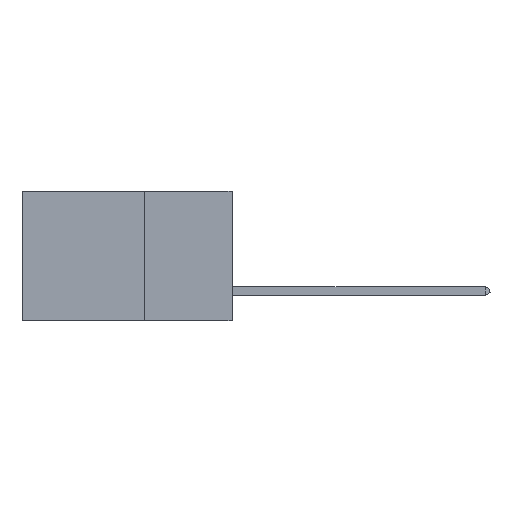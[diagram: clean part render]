
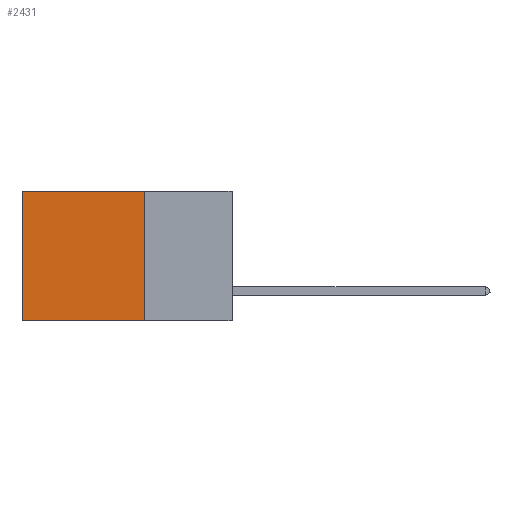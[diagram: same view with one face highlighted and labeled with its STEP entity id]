
A CAD part, left-side view. The second image highlights one B-rep face of the part: STEP entity #2431.
In plain terms, the highlighted planar face has unit normal (-1, 0, 0).
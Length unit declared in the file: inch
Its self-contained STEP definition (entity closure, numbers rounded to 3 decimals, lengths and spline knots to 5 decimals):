
#384 = LINE ( 'NONE', #13258, #7812 ) ;
#436 = CARTESIAN_POINT ( 'NONE',  ( 0.2875, 0.6, 0. ) ) ;
#698 = EDGE_CURVE ( 'NONE', #13443, #2235, #7849, .T. ) ;
#1500 = LINE ( 'NONE', #10485, #12628 ) ;
#2235 = VERTEX_POINT ( 'NONE', #7699 ) ;
#2318 = DIRECTION ( 'NONE',  ( 0., 0., -1. ) ) ;
#2431 = ADVANCED_FACE ( 'NONE', ( #4590 ), #15147, .F. ) ;
#3210 = DIRECTION ( 'NONE',  ( 1., 0., 0. ) ) ;
#4590 = FACE_OUTER_BOUND ( 'NONE', #7172, .T. ) ;
#5385 = VECTOR ( 'NONE', #9371, 39.37008 ) ;
#5554 = CARTESIAN_POINT ( 'NONE',  ( 0.2875, 0.25, 0. ) ) ;
#5984 = DIRECTION ( 'NONE',  ( 0., 0., -1. ) ) ;
#6210 = EDGE_CURVE ( 'NONE', #13443, #13359, #7792, .T. ) ;
#6756 = CARTESIAN_POINT ( 'NONE',  ( 0.2875, 0.25, 0. ) ) ;
#6847 = VERTEX_POINT ( 'NONE', #8153 ) ;
#7172 = EDGE_LOOP ( 'NONE', ( #7451, #11082, #14947, #13836 ) ) ;
#7451 = ORIENTED_EDGE ( 'NONE', *, *, #8029, .T. ) ;
#7699 = CARTESIAN_POINT ( 'NONE',  ( 0.2875, 0.25, -0.37 ) ) ;
#7792 = LINE ( 'NONE', #5554, #5385 ) ;
#7812 = VECTOR ( 'NONE', #12193, 39.37008 ) ;
#7849 = LINE ( 'NONE', #10805, #13765 ) ;
#8029 = EDGE_CURVE ( 'NONE', #13359, #6847, #1500, .T. ) ;
#8153 = CARTESIAN_POINT ( 'NONE',  ( 0.2875, 0.6, -0.37 ) ) ;
#8276 = EDGE_CURVE ( 'NONE', #2235, #6847, #384, .T. ) ;
#9371 = DIRECTION ( 'NONE',  ( 0., 1., 0. ) ) ;
#10423 = AXIS2_PLACEMENT_3D ( 'NONE', #6756, #3210, #2318 ) ;
#10485 = CARTESIAN_POINT ( 'NONE',  ( 0.2875, 0.6, 0. ) ) ;
#10805 = CARTESIAN_POINT ( 'NONE',  ( 0.2875, 0.25, 0. ) ) ;
#11082 = ORIENTED_EDGE ( 'NONE', *, *, #8276, .F. ) ;
#12193 = DIRECTION ( 'NONE',  ( 0., 1., 0. ) ) ;
#12628 = VECTOR ( 'NONE', #12885, 39.37008 ) ;
#12885 = DIRECTION ( 'NONE',  ( 0., 0., -1. ) ) ;
#13007 = CARTESIAN_POINT ( 'NONE',  ( 0.2875, 0.25, 0. ) ) ;
#13258 = CARTESIAN_POINT ( 'NONE',  ( 0.2875, 0.25, -0.37 ) ) ;
#13359 = VERTEX_POINT ( 'NONE', #436 ) ;
#13443 = VERTEX_POINT ( 'NONE', #13007 ) ;
#13765 = VECTOR ( 'NONE', #5984, 39.37008 ) ;
#13836 = ORIENTED_EDGE ( 'NONE', *, *, #6210, .T. ) ;
#14947 = ORIENTED_EDGE ( 'NONE', *, *, #698, .F. ) ;
#15147 = PLANE ( 'NONE',  #10423 ) ;
